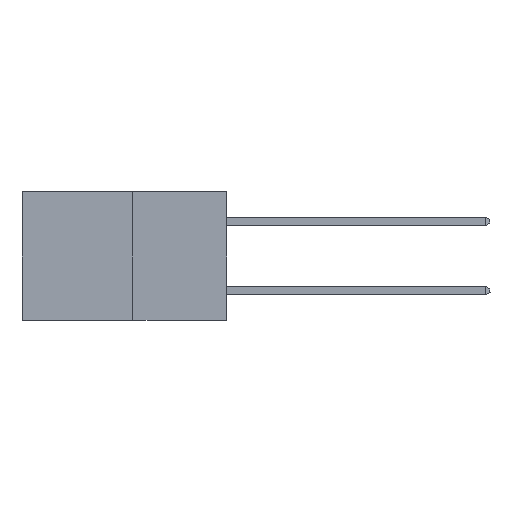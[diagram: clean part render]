
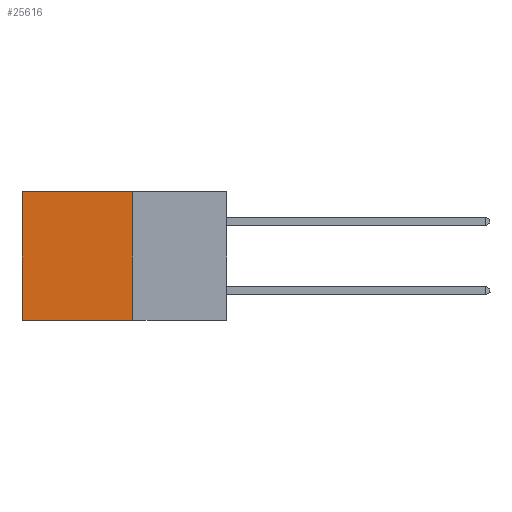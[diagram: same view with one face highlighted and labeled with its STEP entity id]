
A CAD part, left-side view. The second image highlights one B-rep face of the part: STEP entity #25616.
In plain terms, the highlighted planar face has unit normal (-1, 0, 0).
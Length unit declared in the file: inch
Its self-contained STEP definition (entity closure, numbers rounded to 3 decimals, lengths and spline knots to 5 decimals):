
#39 = DIRECTION ( 'NONE',  ( 0., 1., 0. ) ) ;
#939 = CARTESIAN_POINT ( 'NONE',  ( 0.277, 0.59, 0. ) ) ;
#1141 = ORIENTED_EDGE ( 'NONE', *, *, #13186, .F. ) ;
#1546 = AXIS2_PLACEMENT_3D ( 'NONE', #19865, #7327, #21946 ) ;
#3676 = DIRECTION ( 'NONE',  ( 0., 0., -1. ) ) ;
#4759 = VECTOR ( 'NONE', #39, 39.37008 ) ;
#4882 = VECTOR ( 'NONE', #8828, 39.37008 ) ;
#5237 = PLANE ( 'NONE',  #1546 ) ;
#5257 = EDGE_CURVE ( 'NONE', #15901, #12531, #11109, .T. ) ;
#6949 = VECTOR ( 'NONE', #3676, 39.37008 ) ;
#7327 = DIRECTION ( 'NONE',  ( 1., 0., 0. ) ) ;
#8513 = CARTESIAN_POINT ( 'NONE',  ( 0.277, 0.59, -0.37 ) ) ;
#8828 = DIRECTION ( 'NONE',  ( 0., 0., -1. ) ) ;
#9254 = EDGE_CURVE ( 'NONE', #22333, #15901, #24517, .T. ) ;
#11109 = LINE ( 'NONE', #8513, #4882 ) ;
#11348 = VERTEX_POINT ( 'NONE', #19726 ) ;
#11749 = EDGE_CURVE ( 'NONE', #11348, #12531, #15247, .T. ) ;
#12531 = VERTEX_POINT ( 'NONE', #22245 ) ;
#12534 = LINE ( 'NONE', #22409, #6949 ) ;
#13186 = EDGE_CURVE ( 'NONE', #22333, #11348, #12534, .T. ) ;
#15247 = LINE ( 'NONE', #20983, #4759 ) ;
#15267 = DIRECTION ( 'NONE',  ( 0., 1., 0. ) ) ;
#15901 = VERTEX_POINT ( 'NONE', #939 ) ;
#17673 = VECTOR ( 'NONE', #15267, 39.37008 ) ;
#19459 = CARTESIAN_POINT ( 'NONE',  ( 0.277, 0.27, 0. ) ) ;
#19682 = EDGE_LOOP ( 'NONE', ( #25390, #25156, #1141, #21135 ) ) ;
#19726 = CARTESIAN_POINT ( 'NONE',  ( 0.277, 0.27, -0.37 ) ) ;
#19865 = CARTESIAN_POINT ( 'NONE',  ( 0.277, 0.27, -0.37 ) ) ;
#20983 = CARTESIAN_POINT ( 'NONE',  ( 0.277, 0.27, -0.37 ) ) ;
#21118 = CARTESIAN_POINT ( 'NONE',  ( 0.277, 0.27, 0. ) ) ;
#21135 = ORIENTED_EDGE ( 'NONE', *, *, #9254, .T. ) ;
#21946 = DIRECTION ( 'NONE',  ( 0., 0., -1. ) ) ;
#22245 = CARTESIAN_POINT ( 'NONE',  ( 0.277, 0.59, -0.37 ) ) ;
#22333 = VERTEX_POINT ( 'NONE', #21118 ) ;
#22409 = CARTESIAN_POINT ( 'NONE',  ( 0.277, 0.27, -0.37 ) ) ;
#24517 = LINE ( 'NONE', #19459, #17673 ) ;
#25156 = ORIENTED_EDGE ( 'NONE', *, *, #11749, .F. ) ;
#25390 = ORIENTED_EDGE ( 'NONE', *, *, #5257, .T. ) ;
#25473 = FACE_OUTER_BOUND ( 'NONE', #19682, .T. ) ;
#25616 = ADVANCED_FACE ( 'NONE', ( #25473 ), #5237, .F. ) ;
